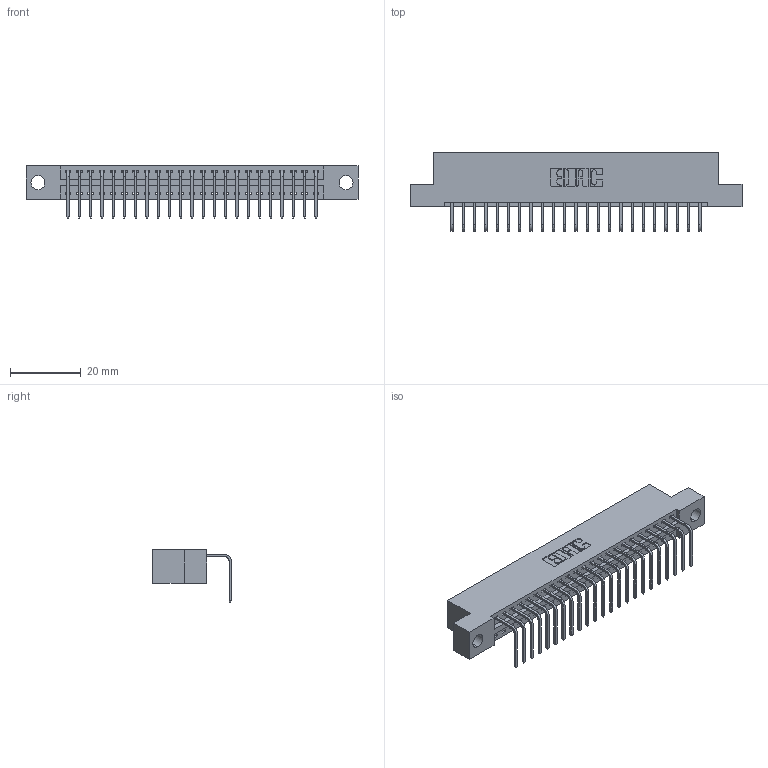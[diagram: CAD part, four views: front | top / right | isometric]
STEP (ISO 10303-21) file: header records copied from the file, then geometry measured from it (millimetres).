
FILE_DESCRIPTION (( 'STEP AP203' ), '1' );
FILE_NAME ('346-023-558-104.STEP', '2022-05-05T21:44:23', ( '' ), ( '' ), 'SwSTEP 2.0', 'SolidWorks 2020', '' );
FILE_SCHEMA (( 'CONFIG_CONTROL_DESIGN' ));
Length unit declared in the file: inch
Products named in the file (3): 345-292-001_558 Tail - 2; 346 Part_Flush Mounting Lugs - 0.156 Dia-TH; 346-023-558-104
Assembly tree (24 placements, depth 2):
  346-023-558-104
    346 Part_Flush Mounting Lugs - 0.156 Dia-TH
    345-292-001_558 Tail - 2  x23
Bounding box: 93.6 x 22.16 x 14.73 mm (x, y, z)
Volume: 8799.3 mm3; surface area: 11087.3 mm2
Topology: 24 solids, 24 shells, 1516 faces, 4551 edges, 3002 vertices
Faces by surface type: plane 1056, cylinder 460
Entity records: 17335 total; most frequent: CARTESIAN_POINT 2987, ORIENTED_EDGE 2942, DIRECTION 2657, EDGE_CURVE 1471, LINE 1247, VECTOR 1247, VERTEX_POINT 978, AXIS2_PLACEMENT_3D 705
